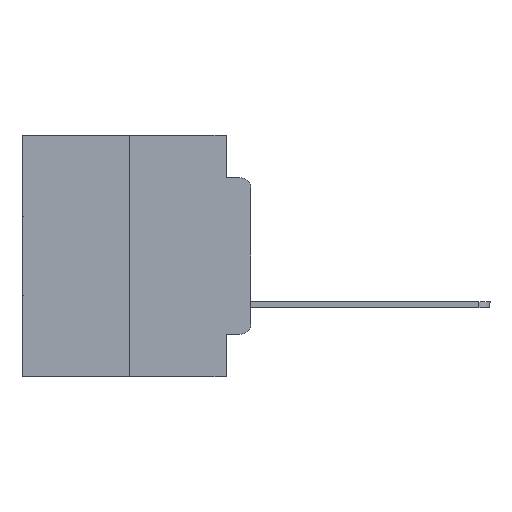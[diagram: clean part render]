
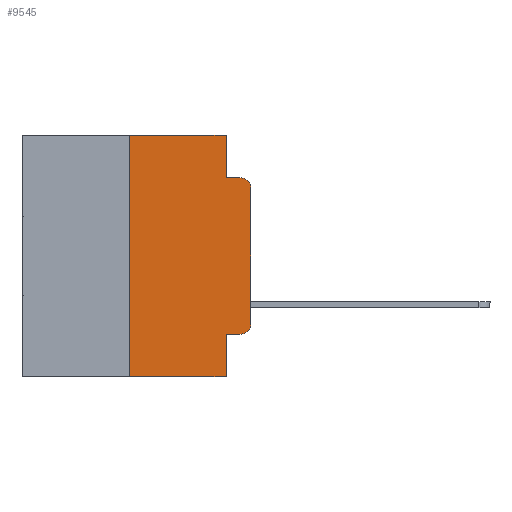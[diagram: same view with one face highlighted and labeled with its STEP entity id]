
A CAD part, left-side view. The second image highlights one B-rep face of the part: STEP entity #9545.
In plain terms, the highlighted planar face has unit normal (-1, 0, 0).
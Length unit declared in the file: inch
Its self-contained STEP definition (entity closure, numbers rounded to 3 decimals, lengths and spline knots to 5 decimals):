
#291 = PLANE ( 'NONE',  #7332 ) ;
#680 = LINE ( 'NONE', #18804, #5073 ) ;
#894 = VERTEX_POINT ( 'NONE', #25342 ) ;
#1274 = EDGE_CURVE ( 'NONE', #24929, #11898, #680, .T. ) ;
#1386 = DIRECTION ( 'NONE',  ( 0., -1., 0. ) ) ;
#1595 = DIRECTION ( 'NONE',  ( 0., 0., -1. ) ) ;
#1796 = ORIENTED_EDGE ( 'NONE', *, *, #16232, .F. ) ;
#2150 = CARTESIAN_POINT ( 'NONE',  ( 0., 0.051, 0. ) ) ;
#2367 = EDGE_CURVE ( 'NONE', #3117, #6214, #28572, .T. ) ;
#2502 = ORIENTED_EDGE ( 'NONE', *, *, #29096, .F. ) ;
#3117 = VERTEX_POINT ( 'NONE', #14233 ) ;
#3761 = LINE ( 'NONE', #10528, #23606 ) ;
#3973 = DIRECTION ( 'NONE',  ( 0., 0., 1. ) ) ;
#4410 = ORIENTED_EDGE ( 'NONE', *, *, #6038, .F. ) ;
#4452 = EDGE_CURVE ( 'NONE', #8421, #894, #3761, .T. ) ;
#4564 = CARTESIAN_POINT ( 'NONE',  ( 0., 0.02, -0.3915 ) ) ;
#5073 = VECTOR ( 'NONE', #16162, 39.37008 ) ;
#5474 = VECTOR ( 'NONE', #27740, 39.37008 ) ;
#5635 = CARTESIAN_POINT ( 'NONE',  ( 0., 0.051, 0. ) ) ;
#6038 = EDGE_CURVE ( 'NONE', #13963, #24929, #16941, .T. ) ;
#6214 = VERTEX_POINT ( 'NONE', #11146 ) ;
#6303 = CARTESIAN_POINT ( 'NONE',  ( 0., 0.051, 0. ) ) ;
#6620 = DIRECTION ( 'NONE',  ( 1., 0., 0. ) ) ;
#6834 = VERTEX_POINT ( 'NONE', #25698 ) ;
#7260 = EDGE_CURVE ( 'NONE', #13963, #9194, #23591, .T. ) ;
#7332 = AXIS2_PLACEMENT_3D ( 'NONE', #18412, #6620, #27099 ) ;
#8176 = EDGE_LOOP ( 'NONE', ( #24993, #15947, #20439, #2502, #15456, #4410, #15900, #1796, #26537, #23887 ) ) ;
#8394 = CARTESIAN_POINT ( 'NONE',  ( 0., 0., 0. ) ) ;
#8421 = VERTEX_POINT ( 'NONE', #19134 ) ;
#9134 = VECTOR ( 'NONE', #25944, 39.37008 ) ;
#9194 = VERTEX_POINT ( 'NONE', #20787 ) ;
#9545 = ADVANCED_FACE ( 'NONE', ( #13681 ), #291, .F. ) ;
#10528 = CARTESIAN_POINT ( 'NONE',  ( 0., 0.051, -0.0885 ) ) ;
#10958 = EDGE_CURVE ( 'NONE', #20425, #3117, #28523, .T. ) ;
#10989 = CARTESIAN_POINT ( 'NONE',  ( 0., 0.02, -0.1085 ) ) ;
#11146 = CARTESIAN_POINT ( 'NONE',  ( 0., 0., -0.1085 ) ) ;
#11446 = LINE ( 'NONE', #6303, #23670 ) ;
#11830 = LINE ( 'NONE', #5635, #5474 ) ;
#11898 = VERTEX_POINT ( 'NONE', #2150 ) ;
#11953 = CARTESIAN_POINT ( 'NONE',  ( 0., 0.473, -0.5 ) ) ;
#12073 = EDGE_CURVE ( 'NONE', #6834, #20425, #21418, .T. ) ;
#12347 = DIRECTION ( 'NONE',  ( 0., 0., 1. ) ) ;
#13681 = FACE_OUTER_BOUND ( 'NONE', #8176, .T. ) ;
#13831 = DIRECTION ( 'NONE',  ( 0., 0., -1. ) ) ;
#13963 = VERTEX_POINT ( 'NONE', #19779 ) ;
#14233 = CARTESIAN_POINT ( 'NONE',  ( 0., 0., -0.3915 ) ) ;
#15456 = ORIENTED_EDGE ( 'NONE', *, *, #1274, .F. ) ;
#15603 = DIRECTION ( 'NONE',  ( 0., 0., -1. ) ) ;
#15839 = AXIS2_PLACEMENT_3D ( 'NONE', #4564, #20470, #13831 ) ;
#15900 = ORIENTED_EDGE ( 'NONE', *, *, #7260, .T. ) ;
#15947 = ORIENTED_EDGE ( 'NONE', *, *, #17410, .T. ) ;
#16055 = VECTOR ( 'NONE', #3973, 39.37008 ) ;
#16162 = DIRECTION ( 'NONE',  ( 0., -1., 0. ) ) ;
#16232 = EDGE_CURVE ( 'NONE', #6834, #9194, #11830, .T. ) ;
#16941 = LINE ( 'NONE', #28404, #17564 ) ;
#17410 = EDGE_CURVE ( 'NONE', #6214, #894, #21538, .T. ) ;
#17564 = VECTOR ( 'NONE', #12347, 39.37008 ) ;
#18412 = CARTESIAN_POINT ( 'NONE',  ( 0., 0.473, 0. ) ) ;
#18495 = CARTESIAN_POINT ( 'NONE',  ( 0., 0.25, 0. ) ) ;
#18804 = CARTESIAN_POINT ( 'NONE',  ( 0., 0.473, 0. ) ) ;
#19134 = CARTESIAN_POINT ( 'NONE',  ( 0., 0.051, -0.0885 ) ) ;
#19779 = CARTESIAN_POINT ( 'NONE',  ( 0., 0.25, -0.5 ) ) ;
#19796 = CARTESIAN_POINT ( 'NONE',  ( 0., 0.051, -0.4115 ) ) ;
#20136 = VECTOR ( 'NONE', #1386, 39.37008 ) ;
#20425 = VERTEX_POINT ( 'NONE', #26456 ) ;
#20439 = ORIENTED_EDGE ( 'NONE', *, *, #4452, .F. ) ;
#20470 = DIRECTION ( 'NONE',  ( -1., 0., 0. ) ) ;
#20787 = CARTESIAN_POINT ( 'NONE',  ( 0., 0.051, -0.5 ) ) ;
#21418 = LINE ( 'NONE', #19796, #20136 ) ;
#21538 = CIRCLE ( 'NONE', #23891, 0.02 ) ;
#23591 = LINE ( 'NONE', #11953, #9134 ) ;
#23606 = VECTOR ( 'NONE', #26295, 39.37008 ) ;
#23670 = VECTOR ( 'NONE', #15603, 39.37008 ) ;
#23887 = ORIENTED_EDGE ( 'NONE', *, *, #10958, .T. ) ;
#23891 = AXIS2_PLACEMENT_3D ( 'NONE', #10989, #28835, #1595 ) ;
#24929 = VERTEX_POINT ( 'NONE', #18495 ) ;
#24993 = ORIENTED_EDGE ( 'NONE', *, *, #2367, .T. ) ;
#25342 = CARTESIAN_POINT ( 'NONE',  ( 0., 0.02, -0.0885 ) ) ;
#25698 = CARTESIAN_POINT ( 'NONE',  ( 0., 0.051, -0.4115 ) ) ;
#25944 = DIRECTION ( 'NONE',  ( 0., -1., 0. ) ) ;
#26295 = DIRECTION ( 'NONE',  ( 0., -1., 0. ) ) ;
#26456 = CARTESIAN_POINT ( 'NONE',  ( 0., 0.02, -0.4115 ) ) ;
#26537 = ORIENTED_EDGE ( 'NONE', *, *, #12073, .T. ) ;
#27099 = DIRECTION ( 'NONE',  ( 0., 0., -1. ) ) ;
#27740 = DIRECTION ( 'NONE',  ( 0., 0., -1. ) ) ;
#28404 = CARTESIAN_POINT ( 'NONE',  ( 0., 0.25, 0. ) ) ;
#28523 = CIRCLE ( 'NONE', #15839, 0.02 ) ;
#28572 = LINE ( 'NONE', #8394, #16055 ) ;
#28835 = DIRECTION ( 'NONE',  ( -1., 0., 0. ) ) ;
#29096 = EDGE_CURVE ( 'NONE', #11898, #8421, #11446, .T. ) ;
